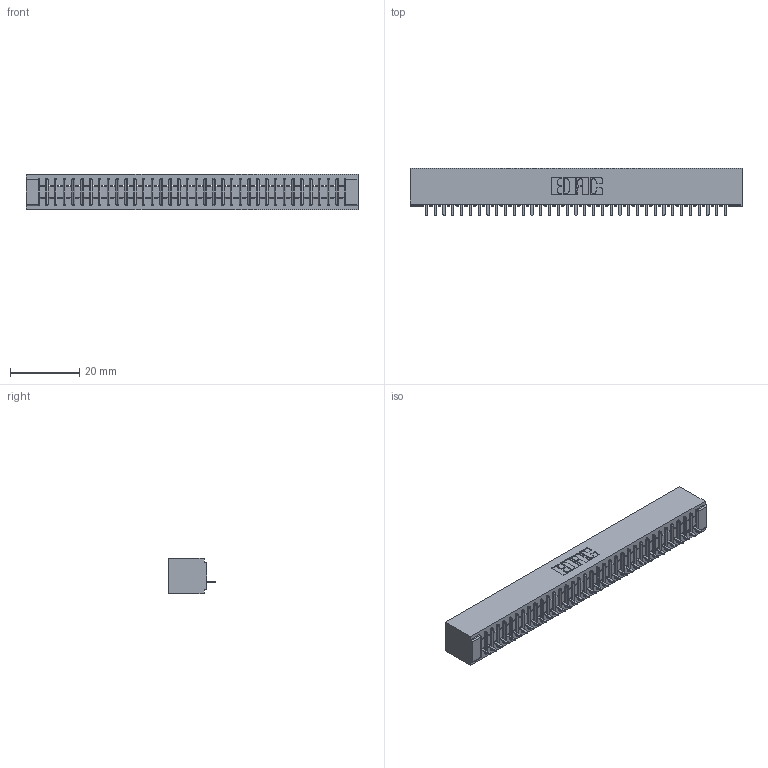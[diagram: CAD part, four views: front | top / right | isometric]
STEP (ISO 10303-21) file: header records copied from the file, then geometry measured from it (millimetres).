
FILE_DESCRIPTION (( 'STEP AP203' ), '1' );
FILE_NAME ('391-035-524-101.STEP', '2018-08-08T23:11:48', ( '' ), ( '' ), 'SwSTEP 2.0', 'SolidWorks 2016', '' );
FILE_SCHEMA (( 'CONFIG_CONTROL_DESIGN' ));
Length unit declared in the file: inch
Products named in the file (3): 341 Part_No Mounting Lugs; 341-292-001_341-292-124; 391-035-524-101
Assembly tree (36 placements, depth 2):
  391-035-524-101
    341 Part_No Mounting Lugs
    341-292-001_341-292-124  x35
Bounding box: 95.89 x 13.64 x 10.16 mm (x, y, z)
Volume: 7056.5 mm3; surface area: 11157.2 mm2
Topology: 36 solids, 36 shells, 2978 faces, 8587 edges, 5510 vertices
Faces by surface type: plane 1849, cylinder 989, sphere 72, torus 68
Entity records: 41892 total; most frequent: CARTESIAN_POINT 7114, ORIENTED_EDGE 7102, DIRECTION 6871, EDGE_CURVE 3551, VECTOR 2865, LINE 2865, VERTEX_POINT 2246, AXIS2_PLACEMENT_3D 2003
